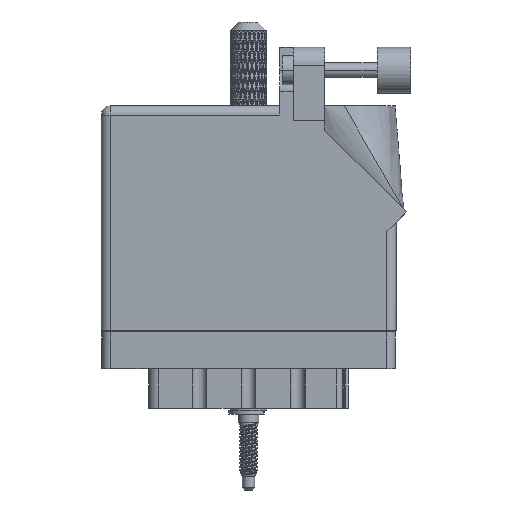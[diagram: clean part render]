
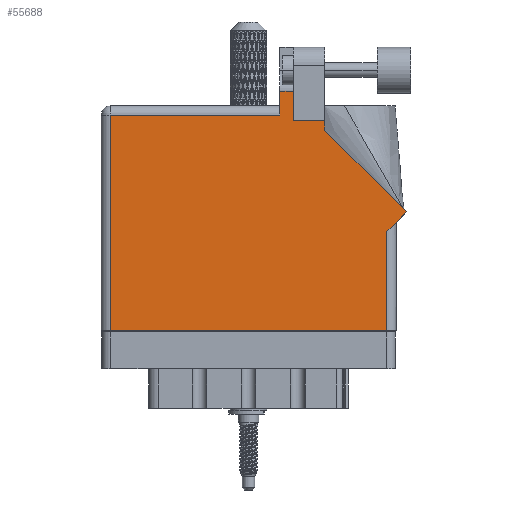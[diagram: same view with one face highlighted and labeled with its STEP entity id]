
A CAD part, front view. The second image highlights one B-rep face of the part: STEP entity #55688.
In plain terms, the highlighted face is planar.
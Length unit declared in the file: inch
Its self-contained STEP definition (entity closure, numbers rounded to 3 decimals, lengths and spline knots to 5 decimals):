
#188 = EDGE_CURVE ( 'NONE', #74149, #95782, #47787, .T. ) ;
#2654 = VECTOR ( 'NONE', #78552, 39.37008 ) ;
#5507 = DIRECTION ( 'NONE',  ( -0.707, 0.707, 0. ) ) ;
#5564 = CARTESIAN_POINT ( 'NONE',  ( 1.948, 0.737, 0. ) ) ;
#7456 = ORIENTED_EDGE ( 'NONE', *, *, #51889, .T. ) ;
#7638 = CARTESIAN_POINT ( 'NONE',  ( 1.217, 1.6315, 0. ) ) ;
#9274 = VECTOR ( 'NONE', #28704, 39.37008 ) ;
#13072 = CARTESIAN_POINT ( 'NONE',  ( 1.217, 1.468, 0. ) ) ;
#14190 = EDGE_CURVE ( 'NONE', #104807, #74149, #14258, .T. ) ;
#14258 = LINE ( 'NONE', #71188, #99757 ) ;
#14503 = CARTESIAN_POINT ( 'NONE',  ( 2.08071, 0.80771, 0. ) ) ;
#14588 = DIRECTION ( 'NONE',  ( -1., 0., 0. ) ) ;
#14829 = VECTOR ( 'NONE', #54721, 39.37008 ) ;
#15816 = CARTESIAN_POINT ( 'NONE',  ( 0.062, 0., 0. ) ) ;
#16315 = CARTESIAN_POINT ( 'NONE',  ( 1.524, 1.43, 0. ) ) ;
#17591 = ORIENTED_EDGE ( 'NONE', *, *, #65644, .T. ) ;
#17906 = EDGE_LOOP ( 'NONE', ( #98813, #32251, #97026, #7456, #22752, #31156, #92721, #88141, #100982, #104082, #17591 ) ) ;
#20072 = CARTESIAN_POINT ( 'NONE',  ( 1.64177, 1.6315, 0. ) ) ;
#21965 = LINE ( 'NONE', #91149, #79021 ) ;
#22752 = ORIENTED_EDGE ( 'NONE', *, *, #68370, .T. ) ;
#23360 = VECTOR ( 'NONE', #5507, 39.37008 ) ;
#24065 = VECTOR ( 'NONE', #58171, 39.37008 ) ;
#24639 = AXIS2_PLACEMENT_3D ( 'NONE', #71121, #72186, #14588 ) ;
#27181 = CARTESIAN_POINT ( 'NONE',  ( 0.062, 1.468, 0. ) ) ;
#28704 = DIRECTION ( 'NONE',  ( 0., 1., 0. ) ) ;
#29524 = VERTEX_POINT ( 'NONE', #100163 ) ;
#29636 = VECTOR ( 'NONE', #63539, 39.37008 ) ;
#30025 = CARTESIAN_POINT ( 'NONE',  ( 0., 1.468, 0. ) ) ;
#31156 = ORIENTED_EDGE ( 'NONE', *, *, #14190, .T. ) ;
#32251 = ORIENTED_EDGE ( 'NONE', *, *, #40735, .T. ) ;
#32483 = LINE ( 'NONE', #30025, #2654 ) ;
#33172 = LINE ( 'NONE', #20072, #49942 ) ;
#34786 = VECTOR ( 'NONE', #84635, 39.37008 ) ;
#37154 = EDGE_CURVE ( 'NONE', #104810, #51605, #102929, .T. ) ;
#40735 = EDGE_CURVE ( 'NONE', #74636, #104810, #33172, .T. ) ;
#44771 = EDGE_CURVE ( 'NONE', #50548, #74636, #105112, .T. ) ;
#47787 = LINE ( 'NONE', #5564, #29636 ) ;
#49942 = VECTOR ( 'NONE', #104051, 39.37008 ) ;
#50548 = VERTEX_POINT ( 'NONE', #60033 ) ;
#51605 = VERTEX_POINT ( 'NONE', #13072 ) ;
#51889 = EDGE_CURVE ( 'NONE', #51605, #71508, #32483, .T. ) ;
#54721 = DIRECTION ( 'NONE',  ( 0., -1., 0. ) ) ;
#55688 = ADVANCED_FACE ( 'NONE', ( #63076 ), #104725, .F. ) ;
#58171 = DIRECTION ( 'NONE',  ( 0., -1., 0. ) ) ;
#59430 = LINE ( 'NONE', #100176, #34786 ) ;
#60033 = CARTESIAN_POINT ( 'NONE',  ( 1.311, 1.43, 0. ) ) ;
#63076 = FACE_OUTER_BOUND ( 'NONE', #17906, .T. ) ;
#63539 = DIRECTION ( 'NONE',  ( 0., 1., 0. ) ) ;
#65644 = EDGE_CURVE ( 'NONE', #102305, #50548, #21965, .T. ) ;
#68370 = EDGE_CURVE ( 'NONE', #71508, #104807, #92808, .T. ) ;
#68683 = CARTESIAN_POINT ( 'NONE',  ( 1.524, 1.36442, 0. ) ) ;
#70008 = CARTESIAN_POINT ( 'NONE',  ( 1.311, 1.43, 0. ) ) ;
#70459 = LINE ( 'NONE', #68683, #78251 ) ;
#71121 = CARTESIAN_POINT ( 'NONE',  ( 0., 1.53, 0. ) ) ;
#71147 = VERTEX_POINT ( 'NONE', #78010 ) ;
#71188 = CARTESIAN_POINT ( 'NONE',  ( 0., 0., 0. ) ) ;
#71508 = VERTEX_POINT ( 'NONE', #27181 ) ;
#72186 = DIRECTION ( 'NONE',  ( 0., 0., -1. ) ) ;
#74149 = VERTEX_POINT ( 'NONE', #98349 ) ;
#74636 = VERTEX_POINT ( 'NONE', #88738 ) ;
#78010 = CARTESIAN_POINT ( 'NONE',  ( 1.524, 1.36442, 0. ) ) ;
#78251 = VECTOR ( 'NONE', #84583, 39.37008 ) ;
#78552 = DIRECTION ( 'NONE',  ( -1., 0., 0. ) ) ;
#79021 = VECTOR ( 'NONE', #99472, 39.37008 ) ;
#80310 = LINE ( 'NONE', #14503, #23360 ) ;
#84583 = DIRECTION ( 'NONE',  ( 0., 1., 0. ) ) ;
#84635 = DIRECTION ( 'NONE',  ( 0.707, 0.707, 0. ) ) ;
#85885 = EDGE_CURVE ( 'NONE', #71147, #102305, #70459, .T. ) ;
#88141 = ORIENTED_EDGE ( 'NONE', *, *, #106092, .T. ) ;
#88738 = CARTESIAN_POINT ( 'NONE',  ( 1.311, 1.6315, 0. ) ) ;
#88918 = DIRECTION ( 'NONE',  ( 1., 0., 0. ) ) ;
#89889 = CARTESIAN_POINT ( 'NONE',  ( 1.948, 0.675, 0. ) ) ;
#91149 = CARTESIAN_POINT ( 'NONE',  ( 1.524, 1.43, 0. ) ) ;
#92721 = ORIENTED_EDGE ( 'NONE', *, *, #188, .T. ) ;
#92808 = LINE ( 'NONE', #15816, #24065 ) ;
#94593 = CARTESIAN_POINT ( 'NONE',  ( 1.217, 1.53, 0. ) ) ;
#95782 = VERTEX_POINT ( 'NONE', #89889 ) ;
#97026 = ORIENTED_EDGE ( 'NONE', *, *, #37154, .T. ) ;
#97120 = CARTESIAN_POINT ( 'NONE',  ( 0.062, 0., 0. ) ) ;
#98349 = CARTESIAN_POINT ( 'NONE',  ( 1.948, 0., 0. ) ) ;
#98813 = ORIENTED_EDGE ( 'NONE', *, *, #44771, .T. ) ;
#99472 = DIRECTION ( 'NONE',  ( -1., 0., 0. ) ) ;
#99757 = VECTOR ( 'NONE', #88918, 39.37008 ) ;
#100163 = CARTESIAN_POINT ( 'NONE',  ( 2.08071, 0.80771, 0. ) ) ;
#100176 = CARTESIAN_POINT ( 'NONE',  ( 2.01, 0.737, 0. ) ) ;
#100982 = ORIENTED_EDGE ( 'NONE', *, *, #104714, .T. ) ;
#102305 = VERTEX_POINT ( 'NONE', #16315 ) ;
#102929 = LINE ( 'NONE', #94593, #14829 ) ;
#104051 = DIRECTION ( 'NONE',  ( -1., 0., 0. ) ) ;
#104082 = ORIENTED_EDGE ( 'NONE', *, *, #85885, .T. ) ;
#104714 = EDGE_CURVE ( 'NONE', #29524, #71147, #80310, .T. ) ;
#104725 = PLANE ( 'NONE',  #24639 ) ;
#104807 = VERTEX_POINT ( 'NONE', #97120 ) ;
#104810 = VERTEX_POINT ( 'NONE', #7638 ) ;
#105112 = LINE ( 'NONE', #70008, #9274 ) ;
#106092 = EDGE_CURVE ( 'NONE', #95782, #29524, #59430, .T. ) ;
